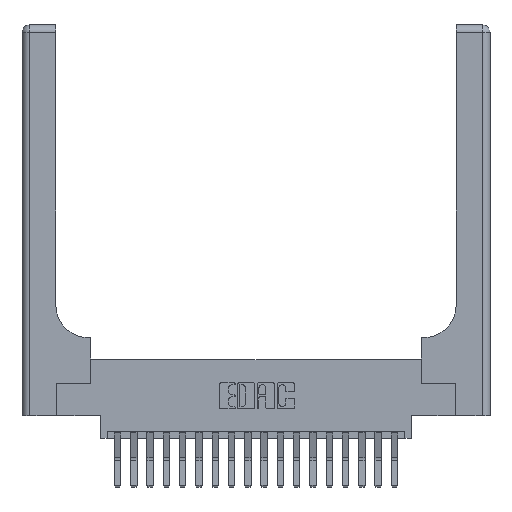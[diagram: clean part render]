
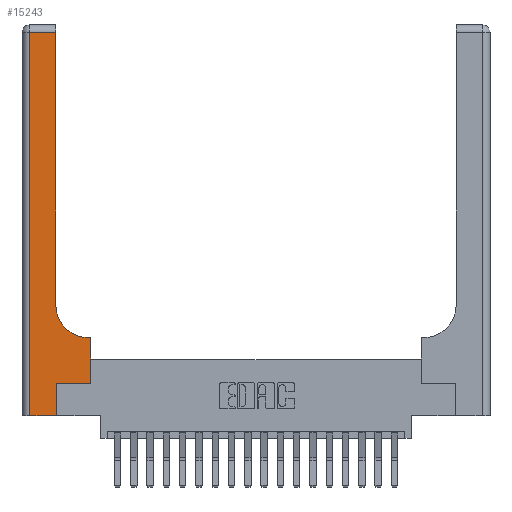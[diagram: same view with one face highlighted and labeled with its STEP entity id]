
A CAD part, top view. The second image highlights one B-rep face of the part: STEP entity #15243.
In plain terms, the highlighted planar face has unit normal (0, 0, 1).
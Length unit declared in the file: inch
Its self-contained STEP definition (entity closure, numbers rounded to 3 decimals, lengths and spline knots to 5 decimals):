
#60 = VERTEX_POINT ( 'NONE', #13018 ) ;
#118 = DIRECTION ( 'NONE',  ( -1., 0., 0. ) ) ;
#222 = LINE ( 'NONE', #15317, #4400 ) ;
#745 = ORIENTED_EDGE ( 'NONE', *, *, #6642, .T. ) ;
#1050 = CIRCLE ( 'NONE', #12800, 0.25 ) ;
#1103 = EDGE_CURVE ( 'NONE', #2886, #1569, #18475, .T. ) ;
#1272 = LINE ( 'NONE', #11831, #9651 ) ;
#1292 = DIRECTION ( 'NONE',  ( 0., 1., 0. ) ) ;
#1400 = ORIENTED_EDGE ( 'NONE', *, *, #6121, .T. ) ;
#1464 = DIRECTION ( 'NONE',  ( 0., -1., 0. ) ) ;
#1469 = EDGE_CURVE ( 'NONE', #11520, #8480, #6881, .T. ) ;
#1524 = LINE ( 'NONE', #15381, #9399 ) ;
#1569 = VERTEX_POINT ( 'NONE', #17420 ) ;
#1606 = DIRECTION ( 'NONE',  ( 1., 0., 0. ) ) ;
#1727 = LINE ( 'NONE', #18876, #9599 ) ;
#1864 = VERTEX_POINT ( 'NONE', #3956 ) ;
#2837 = ORIENTED_EDGE ( 'NONE', *, *, #10328, .T. ) ;
#2886 = VERTEX_POINT ( 'NONE', #11484 ) ;
#3154 = ORIENTED_EDGE ( 'NONE', *, *, #1469, .T. ) ;
#3956 = CARTESIAN_POINT ( 'NONE',  ( 0.51, 0.6, 0.37 ) ) ;
#4158 = CARTESIAN_POINT ( 'NONE',  ( 0., 0., 0.37 ) ) ;
#4238 = ORIENTED_EDGE ( 'NONE', *, *, #1103, .T. ) ;
#4400 = VECTOR ( 'NONE', #16897, 39.37008 ) ;
#5224 = LINE ( 'NONE', #9306, #12631 ) ;
#5651 = DIRECTION ( 'NONE',  ( 1., 0., 0. ) ) ;
#6121 = EDGE_CURVE ( 'NONE', #1864, #6760, #1050, .T. ) ;
#6148 = VECTOR ( 'NONE', #1292, 39.37008 ) ;
#6221 = CARTESIAN_POINT ( 'NONE',  ( 0.51, 0.85, 0.37 ) ) ;
#6580 = EDGE_CURVE ( 'NONE', #8480, #12705, #1524, .T. ) ;
#6642 = EDGE_CURVE ( 'NONE', #60, #11520, #5224, .T. ) ;
#6760 = VERTEX_POINT ( 'NONE', #19023 ) ;
#6881 = LINE ( 'NONE', #4158, #14788 ) ;
#7521 = DIRECTION ( 'NONE',  ( 0., 1., 0. ) ) ;
#7819 = DIRECTION ( 'NONE',  ( 1., 0., 0. ) ) ;
#8019 = CARTESIAN_POINT ( 'NONE',  ( 0.528, 0.25, 0.37 ) ) ;
#8480 = VERTEX_POINT ( 'NONE', #12292 ) ;
#8570 = EDGE_CURVE ( 'NONE', #12705, #2886, #1727, .T. ) ;
#9306 = CARTESIAN_POINT ( 'NONE',  ( 0.06, 3., 0.37 ) ) ;
#9399 = VECTOR ( 'NONE', #7521, 39.37008 ) ;
#9475 = ORIENTED_EDGE ( 'NONE', *, *, #16682, .T. ) ;
#9541 = DIRECTION ( 'NONE',  ( 0., 0., -1. ) ) ;
#9599 = VECTOR ( 'NONE', #1606, 39.37008 ) ;
#9615 = VECTOR ( 'NONE', #11203, 39.37008 ) ;
#9651 = VECTOR ( 'NONE', #13422, 39.37008 ) ;
#10328 = EDGE_CURVE ( 'NONE', #16409, #60, #1272, .T. ) ;
#10605 = ORIENTED_EDGE ( 'NONE', *, *, #18658, .T. ) ;
#11203 = DIRECTION ( 'NONE',  ( 0., 1., 0. ) ) ;
#11484 = CARTESIAN_POINT ( 'NONE',  ( 0.528, 0.25, 0.37 ) ) ;
#11520 = VERTEX_POINT ( 'NONE', #18042 ) ;
#11724 = CARTESIAN_POINT ( 'NONE',  ( 0.26, 2.94, 0.37 ) ) ;
#11831 = CARTESIAN_POINT ( 'NONE',  ( 0., 2.94, 0.37 ) ) ;
#12292 = CARTESIAN_POINT ( 'NONE',  ( 0.265, 0., 0.37 ) ) ;
#12327 = CARTESIAN_POINT ( 'NONE',  ( 0.26, 3., 0.37 ) ) ;
#12631 = VECTOR ( 'NONE', #1464, 39.37008 ) ;
#12705 = VERTEX_POINT ( 'NONE', #17416 ) ;
#12800 = AXIS2_PLACEMENT_3D ( 'NONE', #6221, #17249, #7819 ) ;
#13018 = CARTESIAN_POINT ( 'NONE',  ( 0.06, 2.94, 0.37 ) ) ;
#13422 = DIRECTION ( 'NONE',  ( -1., 0., 0. ) ) ;
#13756 = ORIENTED_EDGE ( 'NONE', *, *, #6580, .T. ) ;
#14228 = CARTESIAN_POINT ( 'NONE',  ( 0., 3., 0.37 ) ) ;
#14788 = VECTOR ( 'NONE', #5651, 39.37008 ) ;
#15129 = ORIENTED_EDGE ( 'NONE', *, *, #8570, .T. ) ;
#15243 = ADVANCED_FACE ( 'NONE', ( #17310 ), #18972, .F. ) ;
#15317 = CARTESIAN_POINT ( 'NONE',  ( 0.26, 0.6, 0.37 ) ) ;
#15381 = CARTESIAN_POINT ( 'NONE',  ( 0.265, 0., 0.37 ) ) ;
#16115 = AXIS2_PLACEMENT_3D ( 'NONE', #14228, #9541, #118 ) ;
#16409 = VERTEX_POINT ( 'NONE', #11724 ) ;
#16682 = EDGE_CURVE ( 'NONE', #6760, #16409, #18521, .T. ) ;
#16897 = DIRECTION ( 'NONE',  ( -1., 0., 0. ) ) ;
#17249 = DIRECTION ( 'NONE',  ( 0., 0., -1. ) ) ;
#17310 = FACE_OUTER_BOUND ( 'NONE', #18478, .T. ) ;
#17416 = CARTESIAN_POINT ( 'NONE',  ( 0.265, 0.25, 0.37 ) ) ;
#17420 = CARTESIAN_POINT ( 'NONE',  ( 0.528, 0.6, 0.37 ) ) ;
#18042 = CARTESIAN_POINT ( 'NONE',  ( 0.06, 0., 0.37 ) ) ;
#18475 = LINE ( 'NONE', #8019, #9615 ) ;
#18478 = EDGE_LOOP ( 'NONE', ( #9475, #2837, #745, #3154, #13756, #15129, #4238, #10605, #1400 ) ) ;
#18521 = LINE ( 'NONE', #12327, #6148 ) ;
#18658 = EDGE_CURVE ( 'NONE', #1569, #1864, #222, .T. ) ;
#18876 = CARTESIAN_POINT ( 'NONE',  ( 0.265, 0.25, 0.37 ) ) ;
#18972 = PLANE ( 'NONE',  #16115 ) ;
#19023 = CARTESIAN_POINT ( 'NONE',  ( 0.26, 0.85, 0.37 ) ) ;
